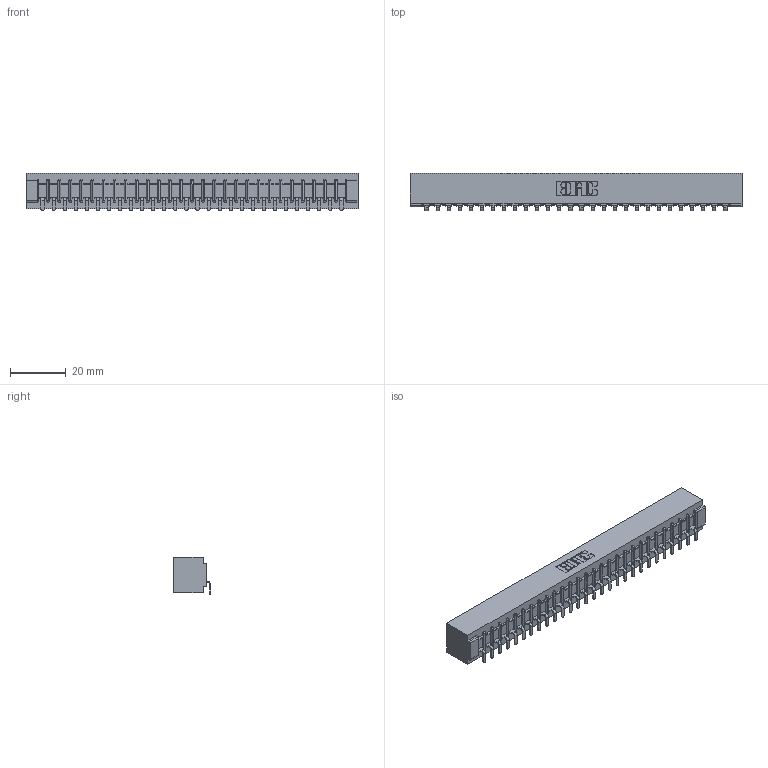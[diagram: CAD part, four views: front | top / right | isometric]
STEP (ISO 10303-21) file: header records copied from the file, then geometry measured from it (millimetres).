
FILE_DESCRIPTION (( 'STEP AP203' ), '1' );
FILE_NAME ('307-028-553-101.STEP', '2019-09-05T03:09:44', ( '' ), ( '' ), 'SwSTEP 2.0', 'SolidWorks 2016', '' );
FILE_SCHEMA (( 'CONFIG_CONTROL_DESIGN' ));
Length unit declared in the file: inch
Products named in the file (3): 307-028-553-101; 307 Part_No Mounting Lugs; 307-290-002_553
Assembly tree (29 placements, depth 2):
  307-028-553-101
    307 Part_No Mounting Lugs
    307-290-002_553  x28
Bounding box: 118.82 x 13.32 x 13.5 mm (x, y, z)
Volume: 13168.6 mm3; surface area: 16596.2 mm2
Topology: 29 solids, 29 shells, 2323 faces, 7131 edges, 4674 vertices
Faces by surface type: plane 1382, cylinder 883, sphere 58
Entity records: 26306 total; most frequent: CARTESIAN_POINT 4436, ORIENTED_EDGE 4426, DIRECTION 4315, EDGE_CURVE 2213, VECTOR 1689, LINE 1689, VERTEX_POINT 1434, AXIS2_PLACEMENT_3D 1313
